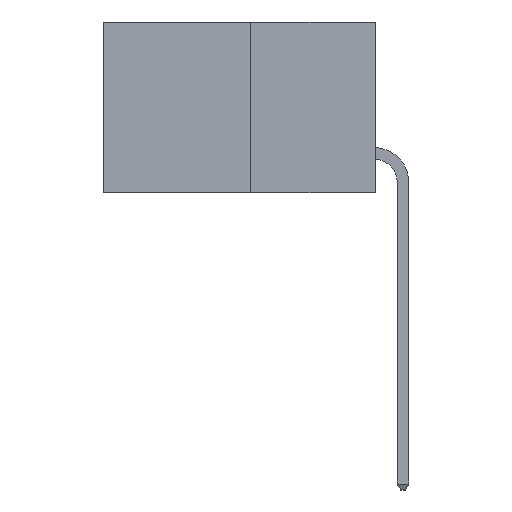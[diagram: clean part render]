
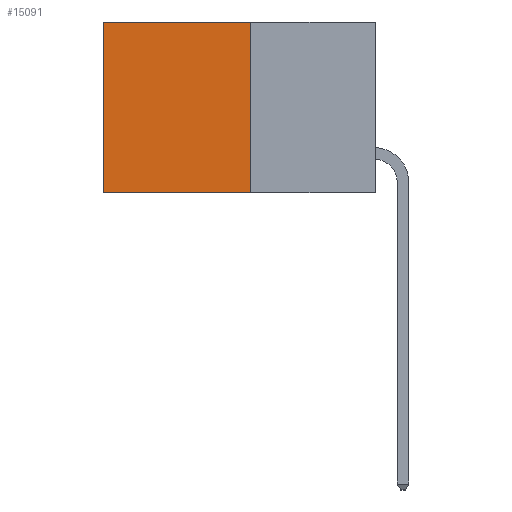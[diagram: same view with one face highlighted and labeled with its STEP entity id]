
A CAD part, left-side view. The second image highlights one B-rep face of the part: STEP entity #15091.
In plain terms, the highlighted planar face has unit normal (-1, 0, 0).
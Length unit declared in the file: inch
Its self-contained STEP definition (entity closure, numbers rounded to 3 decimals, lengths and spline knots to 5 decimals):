
#258 = PLANE ( 'NONE',  #13189 ) ;
#1629 = ORIENTED_EDGE ( 'NONE', *, *, #15183, .F. ) ;
#2494 = CARTESIAN_POINT ( 'NONE',  ( 0.277, 0.59, -0.37 ) ) ;
#2992 = ORIENTED_EDGE ( 'NONE', *, *, #13263, .F. ) ;
#3434 = DIRECTION ( 'NONE',  ( 0., 0., -1. ) ) ;
#3612 = VERTEX_POINT ( 'NONE', #8656 ) ;
#5115 = ORIENTED_EDGE ( 'NONE', *, *, #19072, .T. ) ;
#5330 = EDGE_CURVE ( 'NONE', #14745, #18554, #18804, .T. ) ;
#5569 = FACE_OUTER_BOUND ( 'NONE', #8625, .T. ) ;
#5661 = DIRECTION ( 'NONE',  ( 1., 0., 0. ) ) ;
#8544 = LINE ( 'NONE', #17257, #24555 ) ;
#8625 = EDGE_LOOP ( 'NONE', ( #5115, #2992, #1629, #21772 ) ) ;
#8656 = CARTESIAN_POINT ( 'NONE',  ( 0.277, 0.27, -0.37 ) ) ;
#9071 = CARTESIAN_POINT ( 'NONE',  ( 0.277, 0.27, -0.37 ) ) ;
#10733 = DIRECTION ( 'NONE',  ( 0., 0., -1. ) ) ;
#12582 = VECTOR ( 'NONE', #16466, 39.37008 ) ;
#13168 = VERTEX_POINT ( 'NONE', #2494 ) ;
#13189 = AXIS2_PLACEMENT_3D ( 'NONE', #21242, #5661, #10733 ) ;
#13263 = EDGE_CURVE ( 'NONE', #3612, #13168, #20109, .T. ) ;
#13923 = VECTOR ( 'NONE', #25703, 39.37008 ) ;
#14745 = VERTEX_POINT ( 'NONE', #15906 ) ;
#15091 = ADVANCED_FACE ( 'NONE', ( #5569 ), #258, .F. ) ;
#15183 = EDGE_CURVE ( 'NONE', #14745, #3612, #8544, .T. ) ;
#15906 = CARTESIAN_POINT ( 'NONE',  ( 0.277, 0.27, 0. ) ) ;
#16466 = DIRECTION ( 'NONE',  ( 0., 1., 0. ) ) ;
#17257 = CARTESIAN_POINT ( 'NONE',  ( 0.277, 0.27, -0.37 ) ) ;
#18037 = CARTESIAN_POINT ( 'NONE',  ( 0.277, 0.59, -0.37 ) ) ;
#18554 = VERTEX_POINT ( 'NONE', #18610 ) ;
#18610 = CARTESIAN_POINT ( 'NONE',  ( 0.277, 0.59, 0. ) ) ;
#18777 = VECTOR ( 'NONE', #3434, 39.37008 ) ;
#18804 = LINE ( 'NONE', #19439, #12582 ) ;
#19072 = EDGE_CURVE ( 'NONE', #18554, #13168, #20078, .T. ) ;
#19336 = DIRECTION ( 'NONE',  ( 0., 0., -1. ) ) ;
#19439 = CARTESIAN_POINT ( 'NONE',  ( 0.277, 0.27, 0. ) ) ;
#20078 = LINE ( 'NONE', #18037, #18777 ) ;
#20109 = LINE ( 'NONE', #9071, #13923 ) ;
#21242 = CARTESIAN_POINT ( 'NONE',  ( 0.277, 0.27, -0.37 ) ) ;
#21772 = ORIENTED_EDGE ( 'NONE', *, *, #5330, .T. ) ;
#24555 = VECTOR ( 'NONE', #19336, 39.37008 ) ;
#25703 = DIRECTION ( 'NONE',  ( 0., 1., 0. ) ) ;
